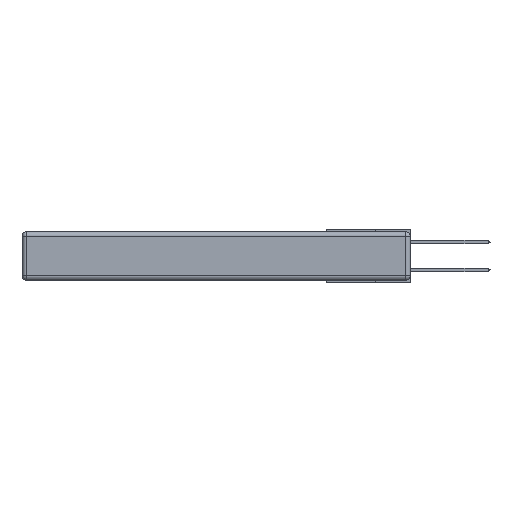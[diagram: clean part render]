
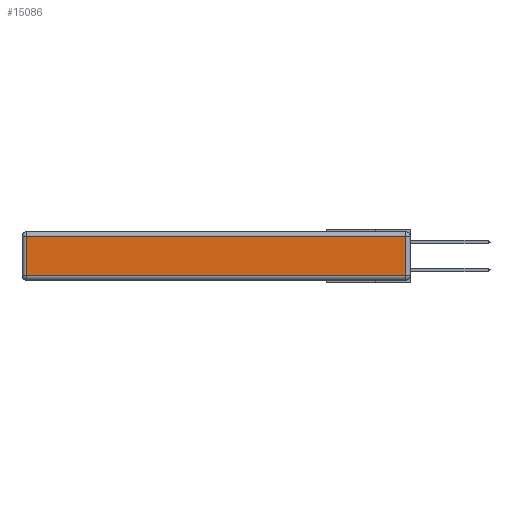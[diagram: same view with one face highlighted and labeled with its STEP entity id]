
A CAD part, left-side view. The second image highlights one B-rep face of the part: STEP entity #15086.
In plain terms, the highlighted planar face has unit normal (-1, 0, 0).
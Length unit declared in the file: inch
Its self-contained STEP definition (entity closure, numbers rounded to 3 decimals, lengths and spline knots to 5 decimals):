
#562 = EDGE_CURVE ( 'NONE', #10332, #3756, #12004, .T. ) ;
#742 = EDGE_CURVE ( 'NONE', #9309, #5003, #18633, .T. ) ;
#944 = CARTESIAN_POINT ( 'NONE',  ( 0., 2.72, -0.343 ) ) ;
#1654 = CARTESIAN_POINT ( 'NONE',  ( 0., 0.03, -0.343 ) ) ;
#2209 = PLANE ( 'NONE',  #16998 ) ;
#3083 = VECTOR ( 'NONE', #3446, 39.37008 ) ;
#3446 = DIRECTION ( 'NONE',  ( 0., 0., 1. ) ) ;
#3756 = VERTEX_POINT ( 'NONE', #20988 ) ;
#4077 = DIRECTION ( 'NONE',  ( -1., 0., 0. ) ) ;
#5003 = VERTEX_POINT ( 'NONE', #5512 ) ;
#5490 = ORIENTED_EDGE ( 'NONE', *, *, #20705, .T. ) ;
#5512 = CARTESIAN_POINT ( 'NONE',  ( 0., 0.03, -0.03 ) ) ;
#6018 = ORIENTED_EDGE ( 'NONE', *, *, #742, .T. ) ;
#6544 = DIRECTION ( 'NONE',  ( 0., 1., 0. ) ) ;
#9125 = FACE_OUTER_BOUND ( 'NONE', #14820, .T. ) ;
#9309 = VERTEX_POINT ( 'NONE', #14059 ) ;
#9982 = CARTESIAN_POINT ( 'NONE',  ( 0., 2.72, -0.03 ) ) ;
#10332 = VERTEX_POINT ( 'NONE', #9982 ) ;
#10644 = CARTESIAN_POINT ( 'NONE',  ( 0., 0., -0.343 ) ) ;
#11000 = LINE ( 'NONE', #11371, #19145 ) ;
#11371 = CARTESIAN_POINT ( 'NONE',  ( 0., 2.75, -0.03 ) ) ;
#11704 = LINE ( 'NONE', #20294, #11943 ) ;
#11943 = VECTOR ( 'NONE', #15224, 39.37008 ) ;
#12004 = LINE ( 'NONE', #944, #13048 ) ;
#12300 = EDGE_CURVE ( 'NONE', #5003, #10332, #11000, .T. ) ;
#12454 = DIRECTION ( 'NONE',  ( 0., 0., -1. ) ) ;
#13048 = VECTOR ( 'NONE', #12454, 39.37008 ) ;
#13361 = ORIENTED_EDGE ( 'NONE', *, *, #12300, .T. ) ;
#14059 = CARTESIAN_POINT ( 'NONE',  ( 0., 0.03, -0.313 ) ) ;
#14820 = EDGE_LOOP ( 'NONE', ( #5490, #6018, #13361, #17936 ) ) ;
#15086 = ADVANCED_FACE ( 'NONE', ( #9125 ), #2209, .T. ) ;
#15224 = DIRECTION ( 'NONE',  ( 0., -1., 0. ) ) ;
#16998 = AXIS2_PLACEMENT_3D ( 'NONE', #10644, #4077, #20185 ) ;
#17936 = ORIENTED_EDGE ( 'NONE', *, *, #562, .T. ) ;
#18633 = LINE ( 'NONE', #1654, #3083 ) ;
#19145 = VECTOR ( 'NONE', #6544, 39.37008 ) ;
#20185 = DIRECTION ( 'NONE',  ( 0., 0., 1. ) ) ;
#20294 = CARTESIAN_POINT ( 'NONE',  ( 0., 0., -0.313 ) ) ;
#20705 = EDGE_CURVE ( 'NONE', #3756, #9309, #11704, .T. ) ;
#20988 = CARTESIAN_POINT ( 'NONE',  ( 0., 2.72, -0.313 ) ) ;
